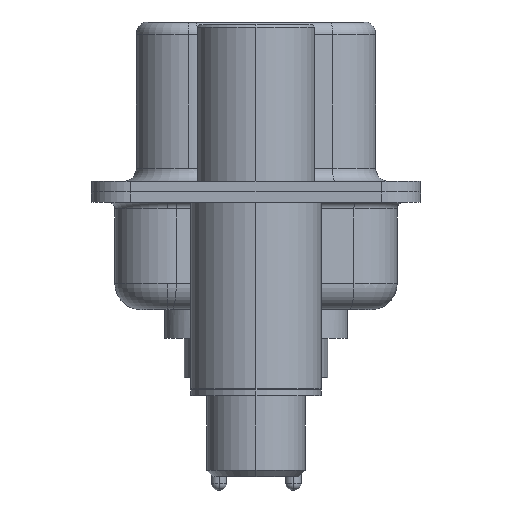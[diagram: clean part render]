
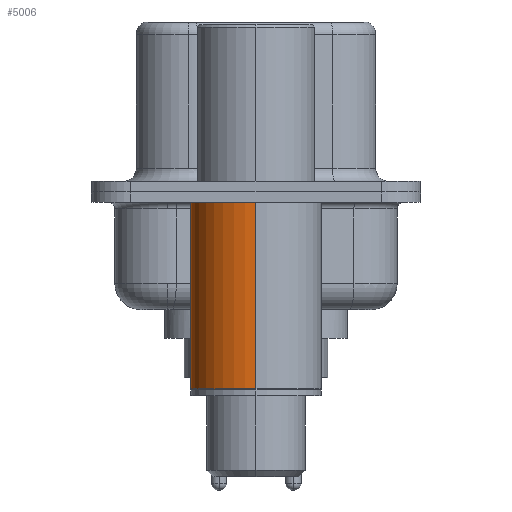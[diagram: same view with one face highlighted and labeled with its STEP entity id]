
A CAD part, left-side view. The second image highlights one B-rep face of the part: STEP entity #5006.
In plain terms, the highlighted cylindrical face has radius 2.5 mm (diameter 5 mm), a partial arc.
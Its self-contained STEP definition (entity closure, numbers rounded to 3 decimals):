
#440 = CARTESIAN_POINT ( 'NONE',  ( -2.5, 0., -7.525 ) ) ;
#574 = ORIENTED_EDGE ( 'NONE', *, *, #15937, .F. ) ;
#957 = ORIENTED_EDGE ( 'NONE', *, *, #15756, .F. ) ;
#1108 = CARTESIAN_POINT ( 'NONE',  ( 0., 0., -7.525 ) ) ;
#1415 = VECTOR ( 'NONE', #9717, 1000. ) ;
#1789 = VERTEX_POINT ( 'NONE', #8027 ) ;
#3331 = CARTESIAN_POINT ( 'NONE',  ( 0., 0., 0.581 ) ) ;
#3382 = DIRECTION ( 'NONE',  ( 1., 0., 0. ) ) ;
#4408 = AXIS2_PLACEMENT_3D ( 'NONE', #1108, #5220, #3382 ) ;
#4477 = DIRECTION ( 'NONE',  ( 0., 0., 1. ) ) ;
#4545 = EDGE_CURVE ( 'NONE', #8910, #11162, #10819, .T. ) ;
#4664 = EDGE_LOOP ( 'NONE', ( #9589, #9139, #957, #574 ) ) ;
#4858 = EDGE_CURVE ( 'NONE', #11162, #1789, #14480, .T. ) ;
#4891 = CARTESIAN_POINT ( 'NONE',  ( 2.5, 0., 0.581 ) ) ;
#5006 = ADVANCED_FACE ( 'NONE', ( #16385 ), #5325, .T. ) ;
#5220 = DIRECTION ( 'NONE',  ( 0., 0., 1. ) ) ;
#5325 = CYLINDRICAL_SURFACE ( 'NONE', #5583, 2.5 ) ;
#5583 = AXIS2_PLACEMENT_3D ( 'NONE', #3331, #16031, #8976 ) ;
#6973 = LINE ( 'NONE', #4891, #17088 ) ;
#8027 = CARTESIAN_POINT ( 'NONE',  ( -2.5, 0., -0.4 ) ) ;
#8910 = VERTEX_POINT ( 'NONE', #10212 ) ;
#8976 = DIRECTION ( 'NONE',  ( 1., 0., 0. ) ) ;
#9139 = ORIENTED_EDGE ( 'NONE', *, *, #4858, .T. ) ;
#9589 = ORIENTED_EDGE ( 'NONE', *, *, #4545, .T. ) ;
#9717 = DIRECTION ( 'NONE',  ( 0., 0., 1. ) ) ;
#10212 = CARTESIAN_POINT ( 'NONE',  ( 2.5, 0., -7.525 ) ) ;
#10225 = DIRECTION ( 'NONE',  ( 0., 0., 1. ) ) ;
#10819 = CIRCLE ( 'NONE', #4408, 2.5 ) ;
#11110 = VERTEX_POINT ( 'NONE', #11302 ) ;
#11162 = VERTEX_POINT ( 'NONE', #440 ) ;
#11302 = CARTESIAN_POINT ( 'NONE',  ( 2.5, 0., -0.4 ) ) ;
#11850 = AXIS2_PLACEMENT_3D ( 'NONE', #12484, #4477, #13806 ) ;
#12484 = CARTESIAN_POINT ( 'NONE',  ( 0., 0., -0.4 ) ) ;
#13806 = DIRECTION ( 'NONE',  ( 1., 0., 0. ) ) ;
#14480 = LINE ( 'NONE', #17354, #1415 ) ;
#15573 = CIRCLE ( 'NONE', #11850, 2.5 ) ;
#15756 = EDGE_CURVE ( 'NONE', #11110, #1789, #15573, .T. ) ;
#15937 = EDGE_CURVE ( 'NONE', #8910, #11110, #6973, .T. ) ;
#16031 = DIRECTION ( 'NONE',  ( 0., 0., 1. ) ) ;
#16385 = FACE_OUTER_BOUND ( 'NONE', #4664, .T. ) ;
#17088 = VECTOR ( 'NONE', #10225, 1000. ) ;
#17354 = CARTESIAN_POINT ( 'NONE',  ( -2.5, 0., 0.581 ) ) ;
